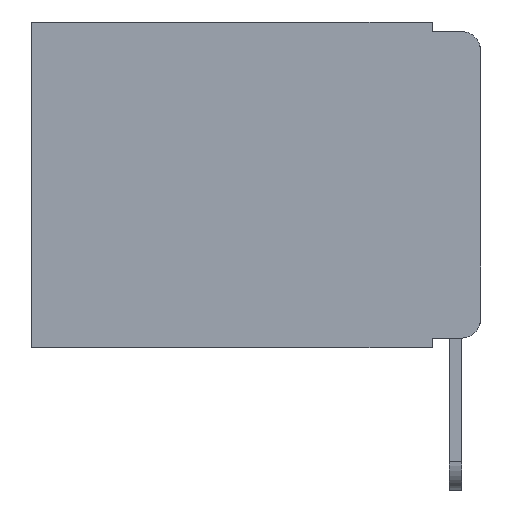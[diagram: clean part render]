
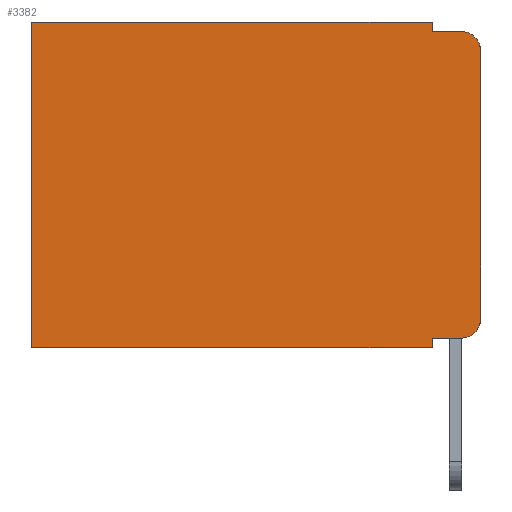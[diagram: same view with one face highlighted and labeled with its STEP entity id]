
A CAD part, left-side view. The second image highlights one B-rep face of the part: STEP entity #3382.
In plain terms, the highlighted planar face has unit normal (-1, 0, 0).
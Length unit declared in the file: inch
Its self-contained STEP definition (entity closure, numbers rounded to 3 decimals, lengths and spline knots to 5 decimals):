
#35 = PLANE ( 'NONE',  #602 ) ;
#81 = CARTESIAN_POINT ( 'NONE',  ( 0.298, 0.051, -0.01 ) ) ;
#419 = ORIENTED_EDGE ( 'NONE', *, *, #3344, .F. ) ;
#456 = DIRECTION ( 'NONE',  ( 0., 0., -1. ) ) ;
#526 = ORIENTED_EDGE ( 'NONE', *, *, #3413, .F. ) ;
#538 = LINE ( 'NONE', #11859, #3248 ) ;
#602 = AXIS2_PLACEMENT_3D ( 'NONE', #10244, #10196, #456 ) ;
#697 = DIRECTION ( 'NONE',  ( 0., 1., 0. ) ) ;
#711 = CIRCLE ( 'NONE', #7388, 0.02 ) ;
#786 = ORIENTED_EDGE ( 'NONE', *, *, #3693, .T. ) ;
#788 = ORIENTED_EDGE ( 'NONE', *, *, #3884, .T. ) ;
#1015 = CARTESIAN_POINT ( 'NONE',  ( 0.298, 0.02, -0.333 ) ) ;
#1072 = ORIENTED_EDGE ( 'NONE', *, *, #3577, .T. ) ;
#1099 = VERTEX_POINT ( 'NONE', #7598 ) ;
#1665 = LINE ( 'NONE', #11895, #9077 ) ;
#1742 = DIRECTION ( 'NONE',  ( 0., 0., -1. ) ) ;
#2016 = CARTESIAN_POINT ( 'NONE',  ( 0.298, 0.473, -0.343 ) ) ;
#2419 = DIRECTION ( 'NONE',  ( 0., 0., -1. ) ) ;
#2549 = LINE ( 'NONE', #5494, #7758 ) ;
#2561 = CARTESIAN_POINT ( 'NONE',  ( 0.298, 0., 0. ) ) ;
#2748 = VECTOR ( 'NONE', #697, 39.37008 ) ;
#2766 = LINE ( 'NONE', #2561, #9921 ) ;
#2857 = EDGE_CURVE ( 'NONE', #1099, #4847, #2766, .T. ) ;
#2987 = EDGE_LOOP ( 'NONE', ( #4361, #4377, #419, #526, #8942, #1072, #5139, #4721, #786, #788 ) ) ;
#3248 = VECTOR ( 'NONE', #11998, 39.37008 ) ;
#3254 = EDGE_CURVE ( 'NONE', #1099, #10131, #711, .T. ) ;
#3344 = EDGE_CURVE ( 'NONE', #4697, #10131, #11324, .T. ) ;
#3382 = ADVANCED_FACE ( 'NONE', ( #10844 ), #35, .F. ) ;
#3413 = EDGE_CURVE ( 'NONE', #11632, #4697, #538, .T. ) ;
#3569 = DIRECTION ( 'NONE',  ( 0., 0., -1. ) ) ;
#3577 = EDGE_CURVE ( 'NONE', #8916, #7417, #1665, .T. ) ;
#3608 = DIRECTION ( 'NONE',  ( -1., 0., 0. ) ) ;
#3633 = EDGE_CURVE ( 'NONE', #10388, #7962, #8791, .T. ) ;
#3669 = CARTESIAN_POINT ( 'NONE',  ( 0.298, 0.02, -0.313 ) ) ;
#3693 = EDGE_CURVE ( 'NONE', #10388, #10928, #2549, .T. ) ;
#3731 = CIRCLE ( 'NONE', #8795, 0.02 ) ;
#3884 = EDGE_CURVE ( 'NONE', #10928, #4847, #3731, .T. ) ;
#4361 = ORIENTED_EDGE ( 'NONE', *, *, #2857, .F. ) ;
#4377 = ORIENTED_EDGE ( 'NONE', *, *, #3254, .T. ) ;
#4676 = EDGE_CURVE ( 'NONE', #11632, #8916, #6631, .T. ) ;
#4697 = VERTEX_POINT ( 'NONE', #9659 ) ;
#4721 = ORIENTED_EDGE ( 'NONE', *, *, #3633, .F. ) ;
#4847 = VERTEX_POINT ( 'NONE', #11528 ) ;
#4862 = CARTESIAN_POINT ( 'NONE',  ( 0.298, 0., -0.343 ) ) ;
#4880 = CARTESIAN_POINT ( 'NONE',  ( 0.298, 0.051, 0. ) ) ;
#5139 = ORIENTED_EDGE ( 'NONE', *, *, #6137, .F. ) ;
#5382 = DIRECTION ( 'NONE',  ( 0., -1., 0. ) ) ;
#5481 = CARTESIAN_POINT ( 'NONE',  ( 0.298, 0.051, 0. ) ) ;
#5494 = CARTESIAN_POINT ( 'NONE',  ( 0.298, 0.051, -0.333 ) ) ;
#5942 = CARTESIAN_POINT ( 'NONE',  ( 0.298, 0.473, 0. ) ) ;
#6137 = EDGE_CURVE ( 'NONE', #7962, #7417, #10188, .T. ) ;
#6631 = LINE ( 'NONE', #11166, #11167 ) ;
#7388 = AXIS2_PLACEMENT_3D ( 'NONE', #8109, #8217, #8196 ) ;
#7417 = VERTEX_POINT ( 'NONE', #2016 ) ;
#7598 = CARTESIAN_POINT ( 'NONE',  ( 0.298, 0., -0.03 ) ) ;
#7758 = VECTOR ( 'NONE', #8025, 39.37008 ) ;
#7816 = DIRECTION ( 'NONE',  ( 0., 1., 0. ) ) ;
#7962 = VERTEX_POINT ( 'NONE', #8409 ) ;
#8025 = DIRECTION ( 'NONE',  ( 0., -1., 0. ) ) ;
#8109 = CARTESIAN_POINT ( 'NONE',  ( 0.298, 0.02, -0.03 ) ) ;
#8196 = DIRECTION ( 'NONE',  ( 0., 0., -1. ) ) ;
#8217 = DIRECTION ( 'NONE',  ( -1., 0., 0. ) ) ;
#8409 = CARTESIAN_POINT ( 'NONE',  ( 0.298, 0.051, -0.343 ) ) ;
#8791 = LINE ( 'NONE', #4880, #10576 ) ;
#8795 = AXIS2_PLACEMENT_3D ( 'NONE', #3669, #3608, #3569 ) ;
#8916 = VERTEX_POINT ( 'NONE', #5942 ) ;
#8942 = ORIENTED_EDGE ( 'NONE', *, *, #4676, .T. ) ;
#9077 = VECTOR ( 'NONE', #10181, 39.37008 ) ;
#9106 = CARTESIAN_POINT ( 'NONE',  ( 0.298, 0.051, -0.333 ) ) ;
#9585 = CARTESIAN_POINT ( 'NONE',  ( 0.298, 0.02, -0.01 ) ) ;
#9659 = CARTESIAN_POINT ( 'NONE',  ( 0.298, 0.051, -0.01 ) ) ;
#9921 = VECTOR ( 'NONE', #1742, 39.37008 ) ;
#10131 = VERTEX_POINT ( 'NONE', #9585 ) ;
#10181 = DIRECTION ( 'NONE',  ( 0., 0., -1. ) ) ;
#10188 = LINE ( 'NONE', #4862, #2748 ) ;
#10196 = DIRECTION ( 'NONE',  ( 1., 0., 0. ) ) ;
#10244 = CARTESIAN_POINT ( 'NONE',  ( 0.298, 0., 0. ) ) ;
#10388 = VERTEX_POINT ( 'NONE', #9106 ) ;
#10576 = VECTOR ( 'NONE', #2419, 39.37008 ) ;
#10844 = FACE_OUTER_BOUND ( 'NONE', #2987, .T. ) ;
#10928 = VERTEX_POINT ( 'NONE', #1015 ) ;
#11166 = CARTESIAN_POINT ( 'NONE',  ( 0.298, 0., 0. ) ) ;
#11167 = VECTOR ( 'NONE', #7816, 39.37008 ) ;
#11324 = LINE ( 'NONE', #81, #12030 ) ;
#11528 = CARTESIAN_POINT ( 'NONE',  ( 0.298, 0., -0.313 ) ) ;
#11632 = VERTEX_POINT ( 'NONE', #5481 ) ;
#11859 = CARTESIAN_POINT ( 'NONE',  ( 0.298, 0.051, 0. ) ) ;
#11895 = CARTESIAN_POINT ( 'NONE',  ( 0.298, 0.473, 0. ) ) ;
#11998 = DIRECTION ( 'NONE',  ( 0., 0., -1. ) ) ;
#12030 = VECTOR ( 'NONE', #5382, 39.37008 ) ;
